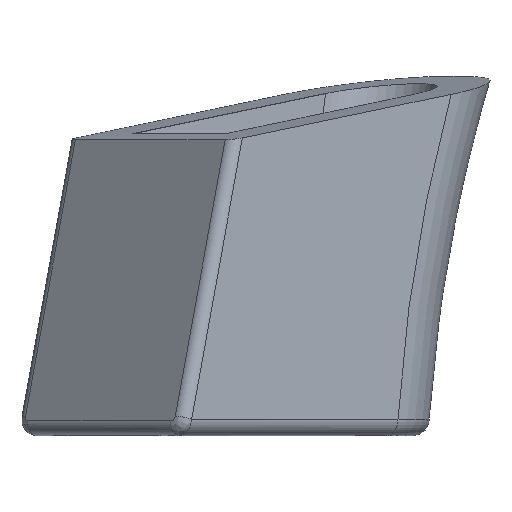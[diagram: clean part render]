
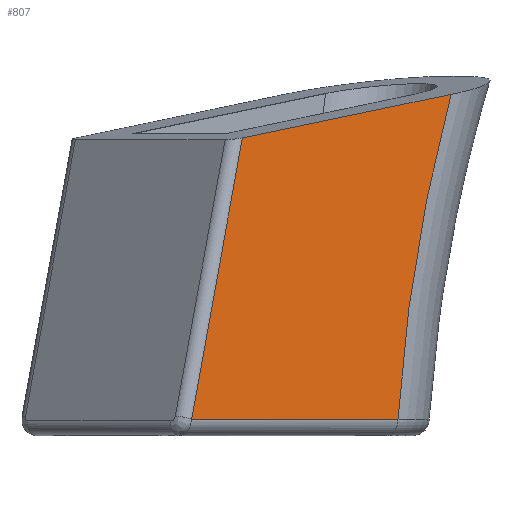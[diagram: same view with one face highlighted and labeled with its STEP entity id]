
A CAD part, front view. The second image highlights one B-rep face of the part: STEP entity #807.
In plain terms, the highlighted planar face has unit normal (0.707, -0.707, 0).
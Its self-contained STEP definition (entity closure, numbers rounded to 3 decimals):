
#40=B_SPLINE_CURVE_WITH_KNOTS('',3,(#1532,#1533,#1534,#1535,#1536,#1537,
#1538,#1539,#1540,#1541,#1542,#1543),.UNSPECIFIED.,.F.,.F.,(4,1,1,1,1,1,
1,1,1,4),(0.,7.693,11.539,15.386,
19.232,23.079,26.925,30.772,34.618,
36.09),.UNSPECIFIED.);
#123=FACE_OUTER_BOUND('',#170,.T.);
#170=EDGE_LOOP('',(#644,#645,#646,#647));
#233=LINE('',#1204,#296);
#241=LINE('',#1300,#304);
#248=LINE('',#1531,#311);
#296=VECTOR('',#994,10.);
#304=VECTOR('',#1016,1.);
#311=VECTOR('',#1033,1.);
#352=VERTEX_POINT('',#1201);
#353=VERTEX_POINT('',#1203);
#361=VERTEX_POINT('',#1298);
#371=VERTEX_POINT('',#1530);
#443=EDGE_CURVE('',#353,#352,#233,.T.);
#457=EDGE_CURVE('',#352,#361,#241,.T.);
#470=EDGE_CURVE('',#361,#371,#248,.T.);
#471=EDGE_CURVE('',#371,#353,#40,.T.);
#644=ORIENTED_EDGE('',*,*,#443,.T.);
#645=ORIENTED_EDGE('',*,*,#457,.T.);
#646=ORIENTED_EDGE('',*,*,#470,.T.);
#647=ORIENTED_EDGE('',*,*,#471,.T.);
#780=PLANE('',#876);
#807=ADVANCED_FACE('',(#123),#780,.F.);
#876=AXIS2_PLACEMENT_3D('',#1529,#1031,#1032);
#994=DIRECTION('',(-0.7,-0.7,-0.146));
#1016=DIRECTION('',(-0.175,-0.175,-0.969));
#1031=DIRECTION('center_axis',(-0.707,0.707,0.));
#1032=DIRECTION('ref_axis',(0.,0.,1.));
#1033=DIRECTION('',(0.707,0.707,0.));
#1201=CARTESIAN_POINT('',(2759.415,287.301,324.67));
#1203=CARTESIAN_POINT('',(2781.941,309.826,329.374));
#1204=CARTESIAN_POINT('',(2775.552,303.438,328.04));
#1298=CARTESIAN_POINT('',(2753.931,281.816,294.318));
#1300=CARTESIAN_POINT('',(2753.931,281.816,294.318));
#1529=CARTESIAN_POINT('Origin',(2773.741,301.626,379.541));
#1530=CARTESIAN_POINT('',(2776.206,304.091,294.318));
#1531=CARTESIAN_POINT('',(2776.206,304.091,294.318));
#1532=CARTESIAN_POINT('Ctrl Pts',(2776.206,304.091,294.318));
#1533=CARTESIAN_POINT('Ctrl Pts',(2776.374,304.259,296.871));
#1534=CARTESIAN_POINT('Ctrl Pts',(2776.703,304.588,300.691));
#1535=CARTESIAN_POINT('Ctrl Pts',(2777.296,305.182,305.751));
#1536=CARTESIAN_POINT('Ctrl Pts',(2777.818,305.704,309.527));
#1537=CARTESIAN_POINT('Ctrl Pts',(2778.417,306.303,313.28));
#1538=CARTESIAN_POINT('Ctrl Pts',(2779.092,306.977,317.007));
#1539=CARTESIAN_POINT('Ctrl Pts',(2779.842,307.727,320.705));
#1540=CARTESIAN_POINT('Ctrl Pts',(2780.666,308.552,324.371));
#1541=CARTESIAN_POINT('Ctrl Pts',(2781.38,309.266,327.254));
#1542=CARTESIAN_POINT('Ctrl Pts',(2781.818,309.703,328.915));
#1543=CARTESIAN_POINT('Ctrl Pts',(2781.941,309.826,329.374));
